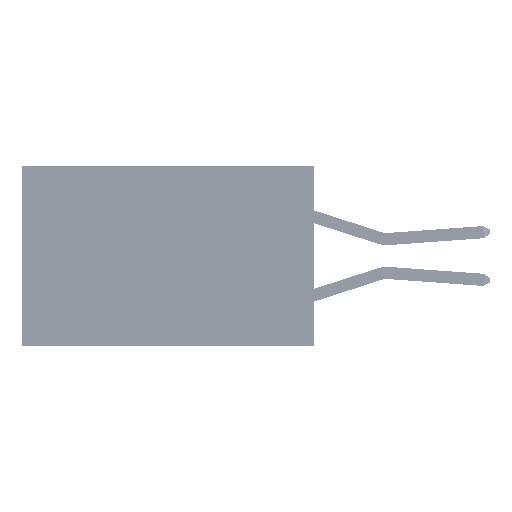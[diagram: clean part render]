
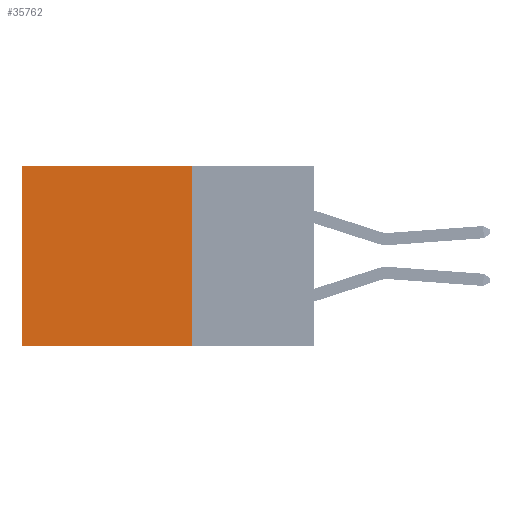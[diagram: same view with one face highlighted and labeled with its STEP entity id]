
A CAD part, left-side view. The second image highlights one B-rep face of the part: STEP entity #35762.
In plain terms, the highlighted planar face has unit normal (-1, 0, 0).
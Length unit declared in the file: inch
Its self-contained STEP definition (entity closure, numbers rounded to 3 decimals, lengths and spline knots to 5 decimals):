
#752 = CARTESIAN_POINT ( 'NONE',  ( 0.2875, 0.6, 0. ) ) ;
#2550 = EDGE_CURVE ( 'NONE', #35086, #3791, #31166, .T. ) ;
#3173 = VECTOR ( 'NONE', #7149, 39.37008 ) ;
#3791 = VERTEX_POINT ( 'NONE', #30917 ) ;
#5644 = EDGE_CURVE ( 'NONE', #11655, #3791, #11801, .T. ) ;
#6044 = ORIENTED_EDGE ( 'NONE', *, *, #50712, .F. ) ;
#7149 = DIRECTION ( 'NONE',  ( 0., 0., -1. ) ) ;
#7580 = CARTESIAN_POINT ( 'NONE',  ( 0.2875, 0.25, 0. ) ) ;
#8951 = DIRECTION ( 'NONE',  ( 0., 0., -1. ) ) ;
#10390 = DIRECTION ( 'NONE',  ( 0., 1., 0. ) ) ;
#11655 = VERTEX_POINT ( 'NONE', #42480 ) ;
#11801 = LINE ( 'NONE', #24316, #48324 ) ;
#12319 = DIRECTION ( 'NONE',  ( 0., 1., 0. ) ) ;
#12390 = CARTESIAN_POINT ( 'NONE',  ( 0.2875, 0.25, 0. ) ) ;
#12873 = PLANE ( 'NONE',  #47810 ) ;
#14198 = EDGE_CURVE ( 'NONE', #48222, #35086, #50138, .T. ) ;
#16327 = CARTESIAN_POINT ( 'NONE',  ( 0.2875, 0.6, 0. ) ) ;
#21491 = DIRECTION ( 'NONE',  ( 0., 0., -1. ) ) ;
#23369 = ORIENTED_EDGE ( 'NONE', *, *, #2550, .T. ) ;
#24316 = CARTESIAN_POINT ( 'NONE',  ( 0.2875, 0.25, -0.37 ) ) ;
#25195 = VECTOR ( 'NONE', #21491, 39.37008 ) ;
#28789 = CARTESIAN_POINT ( 'NONE',  ( 0.2875, 0.25, 0. ) ) ;
#29415 = VECTOR ( 'NONE', #10390, 39.37008 ) ;
#29958 = CARTESIAN_POINT ( 'NONE',  ( 0.2875, 0.25, 0. ) ) ;
#30335 = EDGE_LOOP ( 'NONE', ( #23369, #41459, #6044, #46424 ) ) ;
#30917 = CARTESIAN_POINT ( 'NONE',  ( 0.2875, 0.6, -0.37 ) ) ;
#31166 = LINE ( 'NONE', #752, #3173 ) ;
#35086 = VERTEX_POINT ( 'NONE', #16327 ) ;
#35762 = ADVANCED_FACE ( 'NONE', ( #48712 ), #12873, .F. ) ;
#41390 = LINE ( 'NONE', #12390, #25195 ) ;
#41459 = ORIENTED_EDGE ( 'NONE', *, *, #5644, .F. ) ;
#42480 = CARTESIAN_POINT ( 'NONE',  ( 0.2875, 0.25, -0.37 ) ) ;
#44776 = DIRECTION ( 'NONE',  ( 1., 0., 0. ) ) ;
#46424 = ORIENTED_EDGE ( 'NONE', *, *, #14198, .T. ) ;
#47810 = AXIS2_PLACEMENT_3D ( 'NONE', #28789, #44776, #8951 ) ;
#48222 = VERTEX_POINT ( 'NONE', #7580 ) ;
#48324 = VECTOR ( 'NONE', #12319, 39.37008 ) ;
#48712 = FACE_OUTER_BOUND ( 'NONE', #30335, .T. ) ;
#50138 = LINE ( 'NONE', #29958, #29415 ) ;
#50712 = EDGE_CURVE ( 'NONE', #48222, #11655, #41390, .T. ) ;
